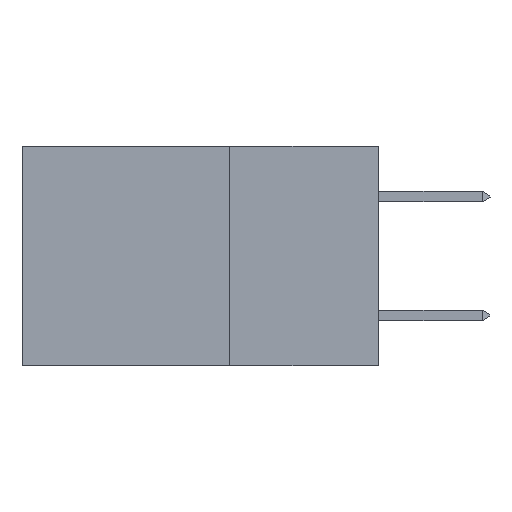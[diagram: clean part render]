
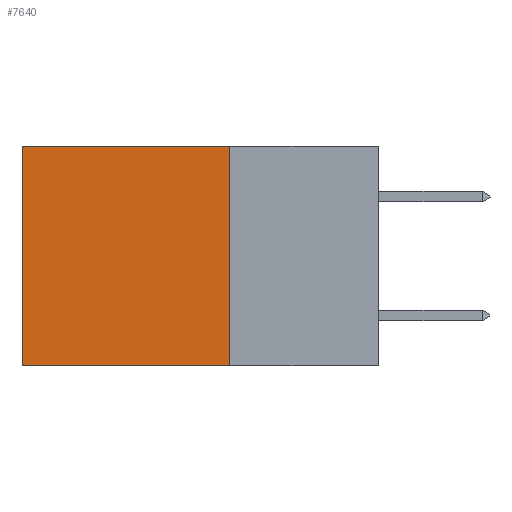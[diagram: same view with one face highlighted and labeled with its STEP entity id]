
A CAD part, left-side view. The second image highlights one B-rep face of the part: STEP entity #7640.
In plain terms, the highlighted planar face has unit normal (-1, 0, 0).
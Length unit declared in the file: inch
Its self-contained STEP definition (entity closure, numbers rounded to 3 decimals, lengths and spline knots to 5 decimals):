
#281 = DIRECTION ( 'NONE',  ( 0., 0., -1. ) ) ;
#703 = VECTOR ( 'NONE', #13846, 39.37008 ) ;
#1231 = LINE ( 'NONE', #5184, #703 ) ;
#1315 = ORIENTED_EDGE ( 'NONE', *, *, #7965, .F. ) ;
#1629 = ORIENTED_EDGE ( 'NONE', *, *, #9249, .T. ) ;
#1816 = AXIS2_PLACEMENT_3D ( 'NONE', #13926, #2966, #6359 ) ;
#2966 = DIRECTION ( 'NONE',  ( 1., 0., 0. ) ) ;
#3291 = CARTESIAN_POINT ( 'NONE',  ( 0.298, 0.25, 0. ) ) ;
#3791 = DIRECTION ( 'NONE',  ( 0., 0., -1. ) ) ;
#4918 = CARTESIAN_POINT ( 'NONE',  ( 0.298, 0.25, 0. ) ) ;
#5184 = CARTESIAN_POINT ( 'NONE',  ( 0.298, 0.25, -0.37 ) ) ;
#5289 = LINE ( 'NONE', #8028, #8009 ) ;
#5700 = FACE_OUTER_BOUND ( 'NONE', #8707, .T. ) ;
#5721 = LINE ( 'NONE', #4918, #12478 ) ;
#6359 = DIRECTION ( 'NONE',  ( 0., 0., -1. ) ) ;
#6372 = CARTESIAN_POINT ( 'NONE',  ( 0.298, 0.6, 0. ) ) ;
#7640 = ADVANCED_FACE ( 'NONE', ( #5700 ), #10342, .F. ) ;
#7771 = VERTEX_POINT ( 'NONE', #3291 ) ;
#7845 = CARTESIAN_POINT ( 'NONE',  ( 0.298, 0.6, -0.37 ) ) ;
#7965 = EDGE_CURVE ( 'NONE', #13173, #9990, #1231, .T. ) ;
#8009 = VECTOR ( 'NONE', #3791, 39.37008 ) ;
#8028 = CARTESIAN_POINT ( 'NONE',  ( 0.298, 0.25, 0. ) ) ;
#8707 = EDGE_LOOP ( 'NONE', ( #1629, #1315, #10644, #9304 ) ) ;
#9249 = EDGE_CURVE ( 'NONE', #11918, #9990, #12257, .T. ) ;
#9304 = ORIENTED_EDGE ( 'NONE', *, *, #12999, .T. ) ;
#9375 = VECTOR ( 'NONE', #281, 39.37008 ) ;
#9990 = VERTEX_POINT ( 'NONE', #7845 ) ;
#10026 = EDGE_CURVE ( 'NONE', #7771, #13173, #5289, .T. ) ;
#10342 = PLANE ( 'NONE',  #1816 ) ;
#10644 = ORIENTED_EDGE ( 'NONE', *, *, #10026, .F. ) ;
#11918 = VERTEX_POINT ( 'NONE', #6372 ) ;
#12257 = LINE ( 'NONE', #13205, #9375 ) ;
#12478 = VECTOR ( 'NONE', #12618, 39.37008 ) ;
#12618 = DIRECTION ( 'NONE',  ( 0., 1., 0. ) ) ;
#12818 = CARTESIAN_POINT ( 'NONE',  ( 0.298, 0.25, -0.37 ) ) ;
#12999 = EDGE_CURVE ( 'NONE', #7771, #11918, #5721, .T. ) ;
#13173 = VERTEX_POINT ( 'NONE', #12818 ) ;
#13205 = CARTESIAN_POINT ( 'NONE',  ( 0.298, 0.6, 0. ) ) ;
#13846 = DIRECTION ( 'NONE',  ( 0., 1., 0. ) ) ;
#13926 = CARTESIAN_POINT ( 'NONE',  ( 0.298, 0.25, 0. ) ) ;
